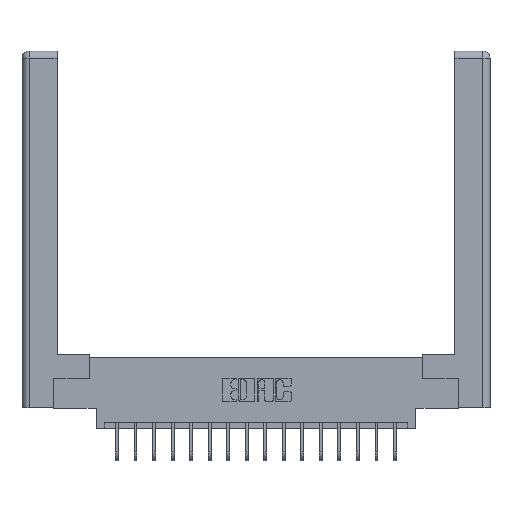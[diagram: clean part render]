
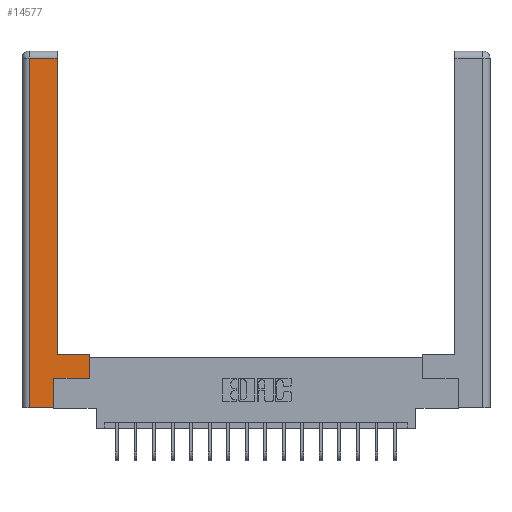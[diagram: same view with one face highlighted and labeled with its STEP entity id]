
A CAD part, top view. The second image highlights one B-rep face of the part: STEP entity #14577.
In plain terms, the highlighted planar face has unit normal (0, 0, 1).
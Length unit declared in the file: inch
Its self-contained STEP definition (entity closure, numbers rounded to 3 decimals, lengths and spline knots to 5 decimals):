
#447 = CARTESIAN_POINT ( 'NONE',  ( 0.265, 0., 0. ) ) ;
#509 = VERTEX_POINT ( 'NONE', #16178 ) ;
#863 = CARTESIAN_POINT ( 'NONE',  ( 0.0615, 0., 0. ) ) ;
#998 = ORIENTED_EDGE ( 'NONE', *, *, #13236, .T. ) ;
#1207 = ORIENTED_EDGE ( 'NONE', *, *, #5307, .T. ) ;
#1264 = ORIENTED_EDGE ( 'NONE', *, *, #1684, .T. ) ;
#1684 = EDGE_CURVE ( 'NONE', #10754, #509, #9922, .T. ) ;
#2444 = DIRECTION ( 'NONE',  ( 0., 1., 0. ) ) ;
#2595 = ORIENTED_EDGE ( 'NONE', *, *, #14700, .T. ) ;
#2674 = CARTESIAN_POINT ( 'NONE',  ( 0.295, 0.45, 0. ) ) ;
#2896 = DIRECTION ( 'NONE',  ( 0., 0., -1. ) ) ;
#2920 = CARTESIAN_POINT ( 'NONE',  ( 0.565, 0.245, 0. ) ) ;
#3459 = CARTESIAN_POINT ( 'NONE',  ( 0.265, 0., 0. ) ) ;
#3613 = LINE ( 'NONE', #863, #18054 ) ;
#3914 = VERTEX_POINT ( 'NONE', #7318 ) ;
#4387 = DIRECTION ( 'NONE',  ( 1., 0., 0. ) ) ;
#4425 = DIRECTION ( 'NONE',  ( 1., 0., 0. ) ) ;
#5044 = VERTEX_POINT ( 'NONE', #10251 ) ;
#5307 = EDGE_CURVE ( 'NONE', #10775, #3914, #8853, .T. ) ;
#5365 = EDGE_CURVE ( 'NONE', #12953, #10775, #11472, .T. ) ;
#5894 = CARTESIAN_POINT ( 'NONE',  ( 0.0615, 0., 0. ) ) ;
#6426 = VECTOR ( 'NONE', #2444, 39.37008 ) ;
#7044 = VECTOR ( 'NONE', #14975, 39.37008 ) ;
#7318 = CARTESIAN_POINT ( 'NONE',  ( 0.295, 2.94, 0. ) ) ;
#7452 = FACE_OUTER_BOUND ( 'NONE', #9002, .T. ) ;
#7915 = VERTEX_POINT ( 'NONE', #3459 ) ;
#8094 = CARTESIAN_POINT ( 'NONE',  ( 0.295, 3., 0. ) ) ;
#8361 = DIRECTION ( 'NONE',  ( -1., 0., 0. ) ) ;
#8482 = CARTESIAN_POINT ( 'NONE',  ( 0., 0., 0. ) ) ;
#8536 = ORIENTED_EDGE ( 'NONE', *, *, #14724, .T. ) ;
#8853 = LINE ( 'NONE', #8094, #6426 ) ;
#9002 = EDGE_LOOP ( 'NONE', ( #1207, #11034, #10592, #2595, #998, #1264, #8536, #11496 ) ) ;
#9226 = LINE ( 'NONE', #14997, #11855 ) ;
#9298 = CARTESIAN_POINT ( 'NONE',  ( 0.0615, 2.94, 0. ) ) ;
#9498 = DIRECTION ( 'NONE',  ( 0., -1., 0. ) ) ;
#9833 = VECTOR ( 'NONE', #4425, 39.37008 ) ;
#9922 = LINE ( 'NONE', #2920, #12102 ) ;
#10153 = VECTOR ( 'NONE', #10904, 39.37008 ) ;
#10251 = CARTESIAN_POINT ( 'NONE',  ( 0.0615, 2.94, 0. ) ) ;
#10592 = ORIENTED_EDGE ( 'NONE', *, *, #15062, .T. ) ;
#10754 = VERTEX_POINT ( 'NONE', #15157 ) ;
#10775 = VERTEX_POINT ( 'NONE', #2674 ) ;
#10904 = DIRECTION ( 'NONE',  ( -1., 0., 0. ) ) ;
#11034 = ORIENTED_EDGE ( 'NONE', *, *, #13841, .T. ) ;
#11291 = PLANE ( 'NONE',  #14594 ) ;
#11472 = LINE ( 'NONE', #13473, #10153 ) ;
#11496 = ORIENTED_EDGE ( 'NONE', *, *, #5365, .T. ) ;
#11855 = VECTOR ( 'NONE', #17852, 39.37008 ) ;
#12102 = VECTOR ( 'NONE', #4387, 39.37008 ) ;
#12677 = CARTESIAN_POINT ( 'NONE',  ( 0.565, 0.45, 0. ) ) ;
#12953 = VERTEX_POINT ( 'NONE', #12677 ) ;
#13236 = EDGE_CURVE ( 'NONE', #7915, #10754, #9226, .T. ) ;
#13473 = CARTESIAN_POINT ( 'NONE',  ( 0.295, 0.45, 0. ) ) ;
#13841 = EDGE_CURVE ( 'NONE', #3914, #5044, #14456, .T. ) ;
#14221 = CARTESIAN_POINT ( 'NONE',  ( 0.565, 0.45, 0. ) ) ;
#14456 = LINE ( 'NONE', #9298, #7044 ) ;
#14577 = ADVANCED_FACE ( 'NONE', ( #7452 ), #11291, .F. ) ;
#14594 = AXIS2_PLACEMENT_3D ( 'NONE', #8482, #2896, #8361 ) ;
#14700 = EDGE_CURVE ( 'NONE', #15851, #7915, #17682, .T. ) ;
#14724 = EDGE_CURVE ( 'NONE', #509, #12953, #15550, .T. ) ;
#14975 = DIRECTION ( 'NONE',  ( -1., 0., 0. ) ) ;
#14997 = CARTESIAN_POINT ( 'NONE',  ( 0.265, 0.245, 0. ) ) ;
#15062 = EDGE_CURVE ( 'NONE', #5044, #15851, #3613, .T. ) ;
#15157 = CARTESIAN_POINT ( 'NONE',  ( 0.265, 0.245, 0. ) ) ;
#15550 = LINE ( 'NONE', #14221, #16403 ) ;
#15599 = DIRECTION ( 'NONE',  ( 0., 1., 0. ) ) ;
#15851 = VERTEX_POINT ( 'NONE', #5894 ) ;
#16178 = CARTESIAN_POINT ( 'NONE',  ( 0.565, 0.245, 0. ) ) ;
#16403 = VECTOR ( 'NONE', #15599, 39.37008 ) ;
#17682 = LINE ( 'NONE', #447, #9833 ) ;
#17852 = DIRECTION ( 'NONE',  ( 0., 1., 0. ) ) ;
#18054 = VECTOR ( 'NONE', #9498, 39.37008 ) ;
